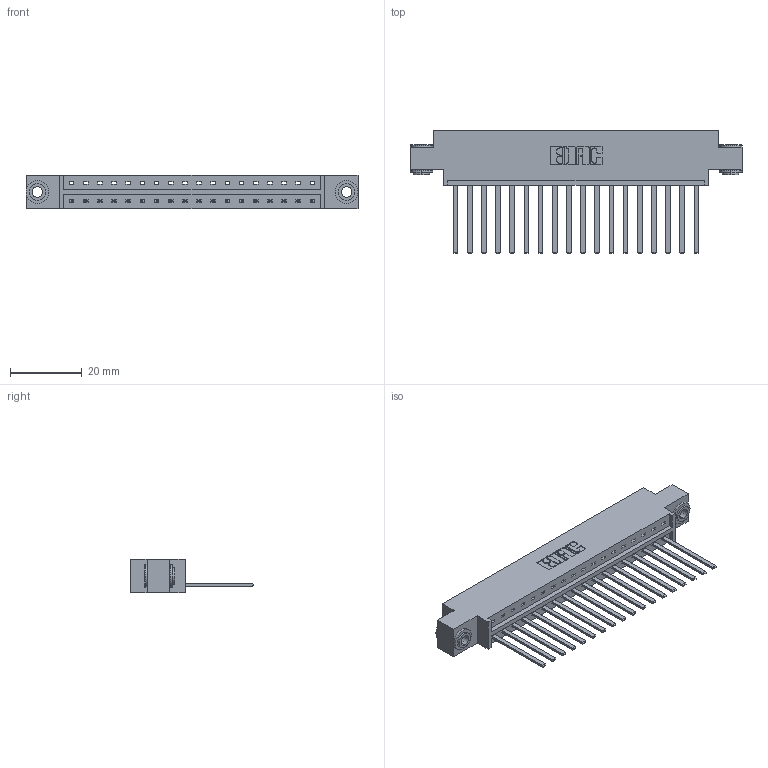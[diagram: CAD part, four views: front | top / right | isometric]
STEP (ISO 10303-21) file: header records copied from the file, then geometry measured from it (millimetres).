
FILE_DESCRIPTION (( 'STEP AP203' ), '1' );
FILE_NAME ('333-018-544-603.STEP', '2019-08-09T13:52:06', ( '' ), ( '' ), 'SwSTEP 2.0', 'SolidWorks 2016', '' );
FILE_SCHEMA (( 'CONFIG_CONTROL_DESIGN' ));
Length unit declared in the file: inch
Products named in the file (4): 333 Part_Offset - .156 Dia - TH; 333-018-544-603; 345-250-002_345-250-002-102; 345-292-001_345-293-144
Assembly tree (21 placements, depth 2):
  333-018-544-603
    333 Part_Offset - .156 Dia - TH
    345-292-001_345-293-144  x18
    345-250-002_345-250-002-102  x2
Bounding box: 92.86 x 34.3 x 9.4 mm (x, y, z)
Volume: 9138.2 mm3; surface area: 10833.7 mm2
Topology: 21 solids, 21 shells, 1092 faces, 3243 edges, 2134 vertices
Faces by surface type: plane 768, cylinder 316, cone 8
Entity records: 14706 total; most frequent: CARTESIAN_POINT 2519, ORIENTED_EDGE 2466, DIRECTION 2203, EDGE_CURVE 1233, VECTOR 1085, LINE 1085, VERTEX_POINT 818, AXIS2_PLACEMENT_3D 559
